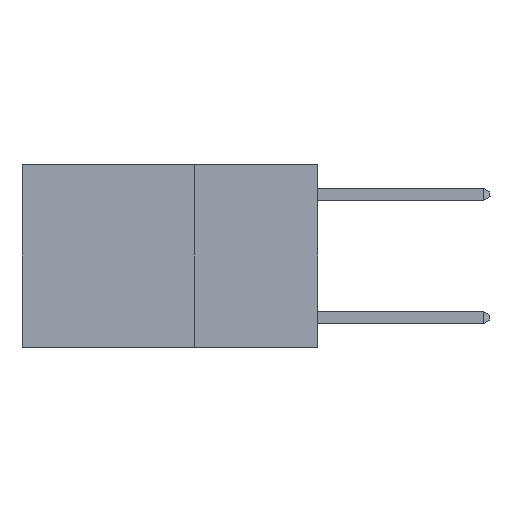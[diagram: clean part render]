
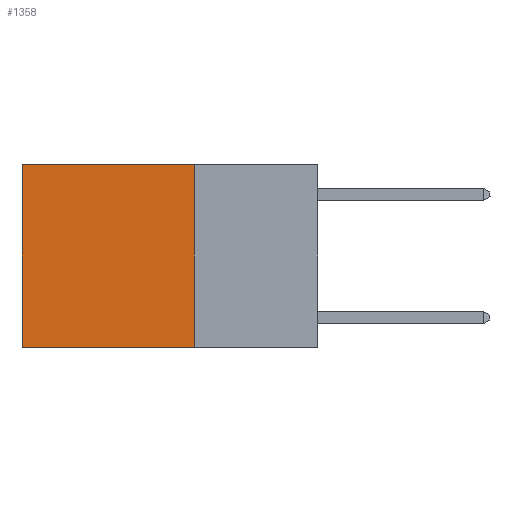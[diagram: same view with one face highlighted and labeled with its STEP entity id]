
A CAD part, left-side view. The second image highlights one B-rep face of the part: STEP entity #1358.
In plain terms, the highlighted planar face has unit normal (-1, 0, 0).
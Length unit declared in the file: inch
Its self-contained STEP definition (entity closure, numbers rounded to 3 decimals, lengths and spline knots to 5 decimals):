
#989 = LINE ( 'NONE', #9834, #7243 ) ;
#1044 = CARTESIAN_POINT ( 'NONE',  ( 0.2625, 0.25, 0. ) ) ;
#1358 = ADVANCED_FACE ( 'NONE', ( #2875 ), #8302, .F. ) ;
#1552 = LINE ( 'NONE', #18279, #4118 ) ;
#1630 = EDGE_CURVE ( 'NONE', #18263, #14548, #989, .T. ) ;
#2046 = VERTEX_POINT ( 'NONE', #19482 ) ;
#2875 = FACE_OUTER_BOUND ( 'NONE', #16829, .T. ) ;
#3384 = DIRECTION ( 'NONE',  ( 0., 0., -1. ) ) ;
#4118 = VECTOR ( 'NONE', #3384, 39.37008 ) ;
#4344 = CARTESIAN_POINT ( 'NONE',  ( 0.2625, 0.25, -0.37 ) ) ;
#4424 = EDGE_CURVE ( 'NONE', #2046, #5529, #20970, .T. ) ;
#5529 = VERTEX_POINT ( 'NONE', #12622 ) ;
#6357 = ORIENTED_EDGE ( 'NONE', *, *, #11060, .T. ) ;
#7243 = VECTOR ( 'NONE', #16870, 39.37008 ) ;
#7428 = ORIENTED_EDGE ( 'NONE', *, *, #1630, .F. ) ;
#8302 = PLANE ( 'NONE',  #15348 ) ;
#8790 = CARTESIAN_POINT ( 'NONE',  ( 0.2625, 0.6, 0. ) ) ;
#8796 = CARTESIAN_POINT ( 'NONE',  ( 0.2625, 0.25, 0. ) ) ;
#8838 = VECTOR ( 'NONE', #15805, 39.37008 ) ;
#9834 = CARTESIAN_POINT ( 'NONE',  ( 0.2625, 0.25, -0.37 ) ) ;
#10162 = DIRECTION ( 'NONE',  ( 0., 1., 0. ) ) ;
#10610 = CARTESIAN_POINT ( 'NONE',  ( 0.2625, 0.6, -0.37 ) ) ;
#11060 = EDGE_CURVE ( 'NONE', #5529, #14548, #14550, .T. ) ;
#12622 = CARTESIAN_POINT ( 'NONE',  ( 0.2625, 0.6, 0. ) ) ;
#14548 = VERTEX_POINT ( 'NONE', #10610 ) ;
#14550 = LINE ( 'NONE', #8790, #8838 ) ;
#14888 = ORIENTED_EDGE ( 'NONE', *, *, #4424, .T. ) ;
#15196 = EDGE_CURVE ( 'NONE', #2046, #18263, #1552, .T. ) ;
#15348 = AXIS2_PLACEMENT_3D ( 'NONE', #1044, #22072, #20473 ) ;
#15794 = ORIENTED_EDGE ( 'NONE', *, *, #15196, .F. ) ;
#15805 = DIRECTION ( 'NONE',  ( 0., 0., -1. ) ) ;
#16829 = EDGE_LOOP ( 'NONE', ( #6357, #7428, #15794, #14888 ) ) ;
#16870 = DIRECTION ( 'NONE',  ( 0., 1., 0. ) ) ;
#18263 = VERTEX_POINT ( 'NONE', #4344 ) ;
#18279 = CARTESIAN_POINT ( 'NONE',  ( 0.2625, 0.25, 0. ) ) ;
#19482 = CARTESIAN_POINT ( 'NONE',  ( 0.2625, 0.25, 0. ) ) ;
#20424 = VECTOR ( 'NONE', #10162, 39.37008 ) ;
#20473 = DIRECTION ( 'NONE',  ( 0., 0., -1. ) ) ;
#20970 = LINE ( 'NONE', #8796, #20424 ) ;
#22072 = DIRECTION ( 'NONE',  ( 1., 0., 0. ) ) ;
